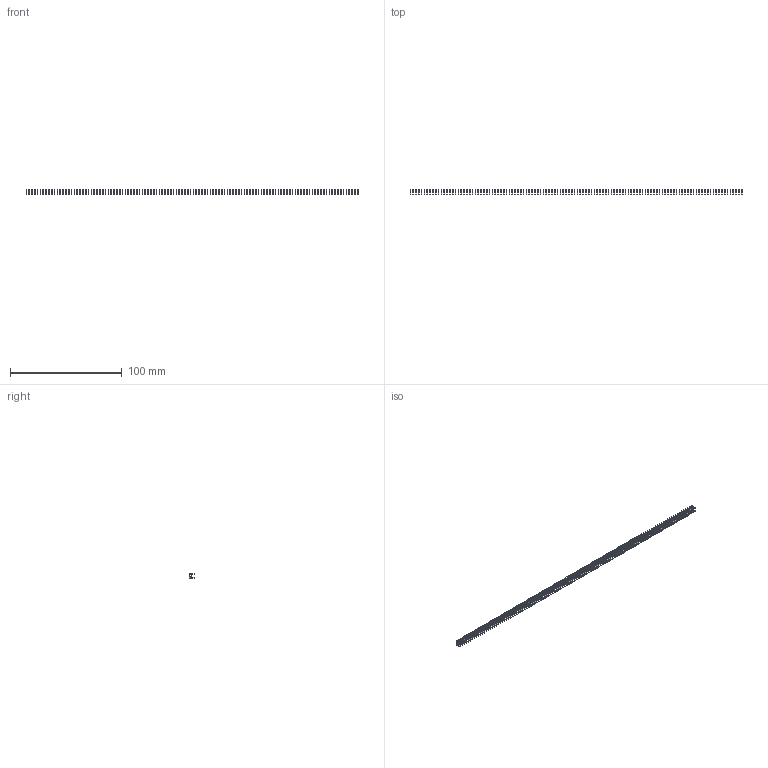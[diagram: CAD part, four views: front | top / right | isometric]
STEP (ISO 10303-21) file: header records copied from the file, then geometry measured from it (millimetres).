
FILE_DESCRIPTION (( 'STEP AP203' ), '1' );
FILE_NAME ('105-118-208-100.STEP', '2020-04-08T01:26:43', ( '' ), ( '' ), 'SwSTEP 2.0', 'SolidWorks 2016', '' );
FILE_SCHEMA (( 'CONFIG_CONTROL_DESIGN' ));
Length unit declared in the file: inch
Products named in the file (2): 105-118-208-100; 100-290-001_100-290-208
Assembly tree (118 placements, depth 2):
  105-118-208-100
    100-290-001_100-290-208  x118
Bounding box: 297.69 x 4.83 x 5.17 mm (x, y, z)
Volume: 811.9 mm3; surface area: 5014.5 mm2
Topology: 118 solids, 118 shells, 2950 faces, 8142 edges, 5428 vertices
Faces by surface type: plane 2596, cylinder 354
Entity records: 4733 total; most frequent: DIRECTION 367, CARTESIAN_POINT 261, CALENDAR_DATE 246, LOCAL_TIME 246, COORDINATED_UNIVERSAL_TIME_OFFSET 246, DATE_AND_TIME 246, AXIS2_PLACEMENT_3D 152, ORIENTED_EDGE 138
